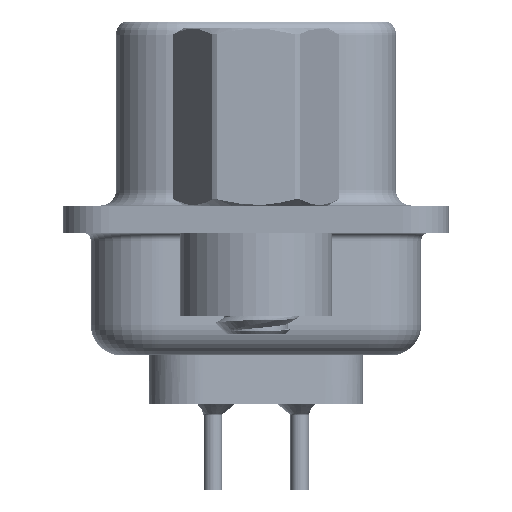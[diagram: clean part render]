
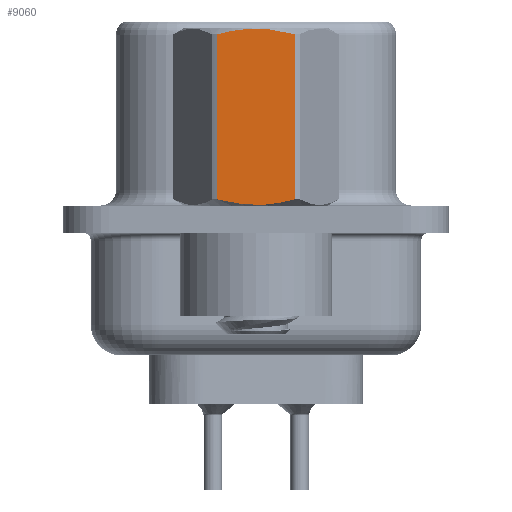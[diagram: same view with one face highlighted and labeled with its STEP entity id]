
A CAD part, left-side view. The second image highlights one B-rep face of the part: STEP entity #9060.
In plain terms, the highlighted planar face has unit normal (-1, 0, 0).
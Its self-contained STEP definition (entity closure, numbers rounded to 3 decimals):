
#518 = CARTESIAN_POINT ( 'NONE',  ( -2.381, 0.428, 6.215 ) ) ;
#1646 = CARTESIAN_POINT ( 'NONE',  ( -2.381, -1.273, 6.048 ) ) ;
#2153 = CARTESIAN_POINT ( 'NONE',  ( -2.381, 0.853, 0.549 ) ) ;
#2187 = B_SPLINE_CURVE_WITH_KNOTS ( 'NONE', 3,
 ( #10865, #5292, #2153, #10030, #5173, #5087, #26973, #27926, #27497, #31047 ),
 .UNSPECIFIED., .F., .F.,
 ( 4, 2, 2, 2, 4 ),
 ( 0.003, 0.003, 0.004, 0.004, 0.005 ),
 .UNSPECIFIED. ) ;
#2473 = B_SPLINE_CURVE_WITH_KNOTS ( 'NONE', 3,
 ( #5731, #11034, #29622, #13708, #32265, #16448, #518, #19131, #3197, #21800 ),
 .UNSPECIFIED., .F., .F.,
 ( 4, 2, 2, 2, 4 ),
 ( 0.001, 0.002, 0.002, 0.003, 0.004 ),
 .UNSPECIFIED. ) ;
#2677 = EDGE_CURVE ( 'NONE', #17719, #20121, #2187, .T. ) ;
#3197 = CARTESIAN_POINT ( 'NONE',  ( -2.381, 1.065, 6.104 ) ) ;
#4870 = VECTOR ( 'NONE', #10588, 1000. ) ;
#5087 = CARTESIAN_POINT ( 'NONE',  ( -2.381, -0.215, 0.468 ) ) ;
#5173 = CARTESIAN_POINT ( 'NONE',  ( -2.381, 0.215, 0.468 ) ) ;
#5292 = CARTESIAN_POINT ( 'NONE',  ( -2.381, 1.065, 0.596 ) ) ;
#5731 = CARTESIAN_POINT ( 'NONE',  ( -2.381, -1.273, 6.048 ) ) ;
#6006 = VECTOR ( 'NONE', #21737, 1000. ) ;
#6490 = VERTEX_POINT ( 'NONE', #10236 ) ;
#8166 = CARTESIAN_POINT ( 'NONE',  ( -2.381, -1.273, 0.652 ) ) ;
#9060 = ADVANCED_FACE ( 'NONE', ( #22626 ), #21110, .T. ) ;
#9564 = AXIS2_PLACEMENT_3D ( 'NONE', #26267, #10439, #29030 ) ;
#10030 = CARTESIAN_POINT ( 'NONE',  ( -2.381, 0.428, 0.485 ) ) ;
#10236 = CARTESIAN_POINT ( 'NONE',  ( -2.381, 1.273, 6.048 ) ) ;
#10319 = EDGE_CURVE ( 'NONE', #20121, #15192, #11880, .T. ) ;
#10439 = DIRECTION ( 'NONE',  ( -1., 0., 0. ) ) ;
#10588 = DIRECTION ( 'NONE',  ( 0., 0., 1. ) ) ;
#10865 = CARTESIAN_POINT ( 'NONE',  ( -2.381, 1.273, 0.652 ) ) ;
#11034 = CARTESIAN_POINT ( 'NONE',  ( -2.381, -1.066, 6.104 ) ) ;
#11684 = EDGE_CURVE ( 'NONE', #6490, #17719, #13898, .T. ) ;
#11880 = LINE ( 'NONE', #21241, #4870 ) ;
#13708 = CARTESIAN_POINT ( 'NONE',  ( -2.381, -0.432, 6.215 ) ) ;
#13778 = CARTESIAN_POINT ( 'NONE',  ( -2.381, 1.273, 3.792 ) ) ;
#13898 = LINE ( 'NONE', #13778, #6006 ) ;
#15192 = VERTEX_POINT ( 'NONE', #1646 ) ;
#16208 = CARTESIAN_POINT ( 'NONE',  ( -2.381, 1.273, 0.652 ) ) ;
#16448 = CARTESIAN_POINT ( 'NONE',  ( -2.381, 0.215, 6.232 ) ) ;
#17719 = VERTEX_POINT ( 'NONE', #16208 ) ;
#19131 = CARTESIAN_POINT ( 'NONE',  ( -2.381, 0.853, 6.151 ) ) ;
#20121 = VERTEX_POINT ( 'NONE', #8166 ) ;
#21110 = PLANE ( 'NONE',  #9564 ) ;
#21241 = CARTESIAN_POINT ( 'NONE',  ( -2.381, -1.273, 3.792 ) ) ;
#21737 = DIRECTION ( 'NONE',  ( 0., 0., -1. ) ) ;
#21800 = CARTESIAN_POINT ( 'NONE',  ( -2.381, 1.273, 6.048 ) ) ;
#22301 = EDGE_LOOP ( 'NONE', ( #33580, #28878, #31802, #30434 ) ) ;
#22626 = FACE_OUTER_BOUND ( 'NONE', #22301, .T. ) ;
#26267 = CARTESIAN_POINT ( 'NONE',  ( -2.381, 1.375, -3.75 ) ) ;
#26973 = CARTESIAN_POINT ( 'NONE',  ( -2.381, -0.432, 0.485 ) ) ;
#27497 = CARTESIAN_POINT ( 'NONE',  ( -2.381, -1.066, 0.596 ) ) ;
#27926 = CARTESIAN_POINT ( 'NONE',  ( -2.381, -0.858, 0.55 ) ) ;
#28878 = ORIENTED_EDGE ( 'NONE', *, *, #10319, .T. ) ;
#29030 = DIRECTION ( 'NONE',  ( 0., -1., 0. ) ) ;
#29622 = CARTESIAN_POINT ( 'NONE',  ( -2.381, -0.858, 6.15 ) ) ;
#30434 = ORIENTED_EDGE ( 'NONE', *, *, #11684, .T. ) ;
#31047 = CARTESIAN_POINT ( 'NONE',  ( -2.381, -1.273, 0.652 ) ) ;
#31802 = ORIENTED_EDGE ( 'NONE', *, *, #33058, .T. ) ;
#32265 = CARTESIAN_POINT ( 'NONE',  ( -2.381, -0.215, 6.232 ) ) ;
#33058 = EDGE_CURVE ( 'NONE', #15192, #6490, #2473, .T. ) ;
#33580 = ORIENTED_EDGE ( 'NONE', *, *, #2677, .T. ) ;
